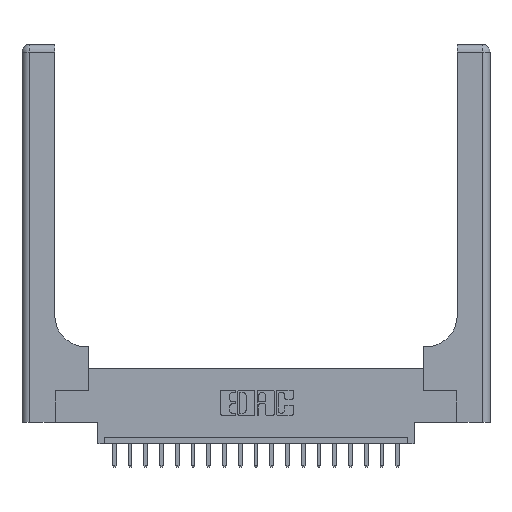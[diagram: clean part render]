
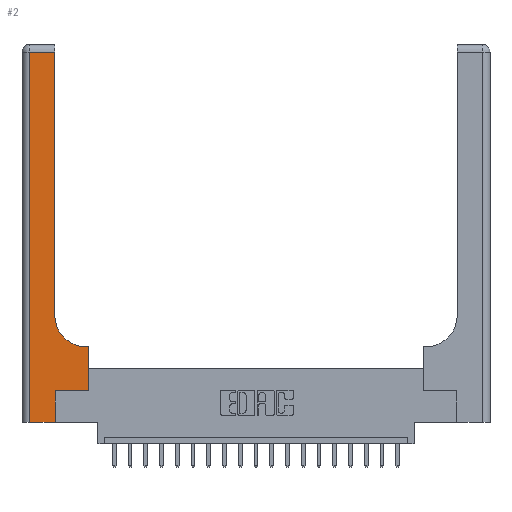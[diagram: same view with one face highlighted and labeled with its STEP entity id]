
A CAD part, top view. The second image highlights one B-rep face of the part: STEP entity #2.
In plain terms, the highlighted planar face has unit normal (0, 0, 1).
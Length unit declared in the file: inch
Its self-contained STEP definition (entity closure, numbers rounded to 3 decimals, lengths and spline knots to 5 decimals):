
#2 = ADVANCED_FACE ( 'NONE', ( #4423 ), #3335, .F. ) ;
#43 = CARTESIAN_POINT ( 'NONE',  ( 0.06, 0., 0.37 ) ) ;
#59 = DIRECTION ( 'NONE',  ( 1., 0., 0. ) ) ;
#412 = VECTOR ( 'NONE', #3590, 39.37008 ) ;
#439 = CARTESIAN_POINT ( 'NONE',  ( 0.528, 0.6, 0.37 ) ) ;
#1073 = CARTESIAN_POINT ( 'NONE',  ( 0.06, 2.94, 0.37 ) ) ;
#1214 = EDGE_CURVE ( 'NONE', #8866, #6385, #16882, .T. ) ;
#1329 = EDGE_CURVE ( 'NONE', #6702, #8866, #7351, .T. ) ;
#1468 = CARTESIAN_POINT ( 'NONE',  ( 0.51, 0.6, 0.37 ) ) ;
#1746 = CARTESIAN_POINT ( 'NONE',  ( 0., 3., 0.37 ) ) ;
#2228 = LINE ( 'NONE', #5715, #3023 ) ;
#2490 = CARTESIAN_POINT ( 'NONE',  ( 0.26, 0.6, 0.37 ) ) ;
#2946 = ORIENTED_EDGE ( 'NONE', *, *, #19983, .T. ) ;
#3023 = VECTOR ( 'NONE', #12104, 39.37008 ) ;
#3148 = CARTESIAN_POINT ( 'NONE',  ( 0.265, 0.25, 0.37 ) ) ;
#3327 = VECTOR ( 'NONE', #11668, 39.37008 ) ;
#3335 = PLANE ( 'NONE',  #8089 ) ;
#3534 = CARTESIAN_POINT ( 'NONE',  ( 0.26, 2.94, 0.37 ) ) ;
#3590 = DIRECTION ( 'NONE',  ( 1., 0., 0. ) ) ;
#3887 = VECTOR ( 'NONE', #16993, 39.37008 ) ;
#3984 = LINE ( 'NONE', #17000, #13377 ) ;
#4297 = DIRECTION ( 'NONE',  ( -1., 0., 0. ) ) ;
#4423 = FACE_OUTER_BOUND ( 'NONE', #15424, .T. ) ;
#5580 = CARTESIAN_POINT ( 'NONE',  ( 0.265, 0.25, 0.37 ) ) ;
#5709 = ORIENTED_EDGE ( 'NONE', *, *, #8388, .T. ) ;
#5715 = CARTESIAN_POINT ( 'NONE',  ( 0., 2.94, 0.37 ) ) ;
#6385 = VERTEX_POINT ( 'NONE', #1468 ) ;
#6392 = DIRECTION ( 'NONE',  ( 0., 0., -1. ) ) ;
#6702 = VERTEX_POINT ( 'NONE', #20242 ) ;
#6704 = EDGE_CURVE ( 'NONE', #16207, #17129, #3984, .T. ) ;
#7351 = LINE ( 'NONE', #18863, #3887 ) ;
#7475 = VERTEX_POINT ( 'NONE', #1073 ) ;
#7934 = CARTESIAN_POINT ( 'NONE',  ( 0.26, 0.85, 0.37 ) ) ;
#8089 = AXIS2_PLACEMENT_3D ( 'NONE', #1746, #20376, #8177 ) ;
#8177 = DIRECTION ( 'NONE',  ( -1., 0., 0. ) ) ;
#8388 = EDGE_CURVE ( 'NONE', #6385, #9327, #10905, .T. ) ;
#8866 = VERTEX_POINT ( 'NONE', #439 ) ;
#9327 = VERTEX_POINT ( 'NONE', #7934 ) ;
#9443 = ORIENTED_EDGE ( 'NONE', *, *, #11903, .T. ) ;
#9516 = CARTESIAN_POINT ( 'NONE',  ( 0.51, 0.85, 0.37 ) ) ;
#9765 = DIRECTION ( 'NONE',  ( 0., 1., 0. ) ) ;
#10229 = AXIS2_PLACEMENT_3D ( 'NONE', #9516, #6392, #59 ) ;
#10452 = ORIENTED_EDGE ( 'NONE', *, *, #16883, .T. ) ;
#10905 = CIRCLE ( 'NONE', #10229, 0.25 ) ;
#10994 = EDGE_CURVE ( 'NONE', #17129, #6702, #18259, .T. ) ;
#11668 = DIRECTION ( 'NONE',  ( 1., 0., 0. ) ) ;
#11903 = EDGE_CURVE ( 'NONE', #17664, #7475, #2228, .T. ) ;
#12104 = DIRECTION ( 'NONE',  ( -1., 0., 0. ) ) ;
#13377 = VECTOR ( 'NONE', #18773, 39.37008 ) ;
#13766 = ORIENTED_EDGE ( 'NONE', *, *, #6704, .T. ) ;
#13805 = ORIENTED_EDGE ( 'NONE', *, *, #10994, .T. ) ;
#14498 = ORIENTED_EDGE ( 'NONE', *, *, #15054, .T. ) ;
#15054 = EDGE_CURVE ( 'NONE', #7475, #18020, #20504, .T. ) ;
#15137 = ORIENTED_EDGE ( 'NONE', *, *, #1214, .T. ) ;
#15424 = EDGE_LOOP ( 'NONE', ( #2946, #9443, #14498, #10452, #13766, #13805, #16739, #15137, #5709 ) ) ;
#15520 = VECTOR ( 'NONE', #20404, 39.37008 ) ;
#15576 = VECTOR ( 'NONE', #4297, 39.37008 ) ;
#15696 = CARTESIAN_POINT ( 'NONE',  ( 0.06, 3., 0.37 ) ) ;
#16207 = VERTEX_POINT ( 'NONE', #20615 ) ;
#16382 = LINE ( 'NONE', #18051, #20629 ) ;
#16739 = ORIENTED_EDGE ( 'NONE', *, *, #1329, .T. ) ;
#16883 = EDGE_CURVE ( 'NONE', #18020, #16207, #17961, .T. ) ;
#16882 = LINE ( 'NONE', #2490, #15576 ) ;
#16993 = DIRECTION ( 'NONE',  ( 0., 1., 0. ) ) ;
#17000 = CARTESIAN_POINT ( 'NONE',  ( 0.265, 0., 0.37 ) ) ;
#17129 = VERTEX_POINT ( 'NONE', #3148 ) ;
#17664 = VERTEX_POINT ( 'NONE', #3534 ) ;
#17961 = LINE ( 'NONE', #19637, #412 ) ;
#18020 = VERTEX_POINT ( 'NONE', #43 ) ;
#18051 = CARTESIAN_POINT ( 'NONE',  ( 0.26, 3., 0.37 ) ) ;
#18259 = LINE ( 'NONE', #5580, #3327 ) ;
#18773 = DIRECTION ( 'NONE',  ( 0., 1., 0. ) ) ;
#18863 = CARTESIAN_POINT ( 'NONE',  ( 0.528, 0.25, 0.37 ) ) ;
#19637 = CARTESIAN_POINT ( 'NONE',  ( 0., 0., 0.37 ) ) ;
#19983 = EDGE_CURVE ( 'NONE', #9327, #17664, #16382, .T. ) ;
#20242 = CARTESIAN_POINT ( 'NONE',  ( 0.528, 0.25, 0.37 ) ) ;
#20376 = DIRECTION ( 'NONE',  ( 0., 0., -1. ) ) ;
#20404 = DIRECTION ( 'NONE',  ( 0., -1., 0. ) ) ;
#20504 = LINE ( 'NONE', #15696, #15520 ) ;
#20615 = CARTESIAN_POINT ( 'NONE',  ( 0.265, 0., 0.37 ) ) ;
#20629 = VECTOR ( 'NONE', #9765, 39.37008 ) ;
